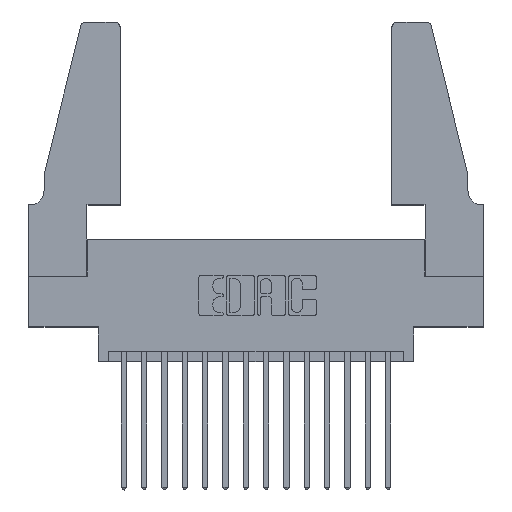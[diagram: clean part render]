
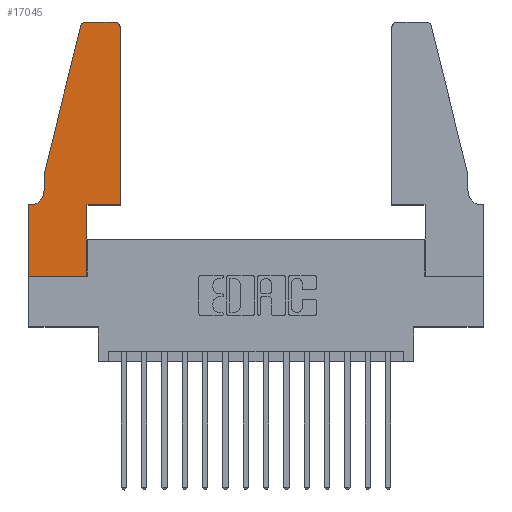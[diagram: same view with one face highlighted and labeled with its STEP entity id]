
A CAD part, top view. The second image highlights one B-rep face of the part: STEP entity #17045.
In plain terms, the highlighted planar face has unit normal (0, 0, 1).
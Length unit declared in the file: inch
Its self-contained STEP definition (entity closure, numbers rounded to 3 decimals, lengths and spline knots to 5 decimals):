
#61 = CARTESIAN_POINT ( 'NONE',  ( 0.284, 1.22, 0.37 ) ) ;
#124 = DIRECTION ( 'NONE',  ( 1., 0., 0. ) ) ;
#344 = EDGE_CURVE ( 'NONE', #13721, #15269, #12927, .T. ) ;
#364 = ORIENTED_EDGE ( 'NONE', *, *, #15349, .T. ) ;
#545 = CIRCLE ( 'NONE', #15114, 0.07 ) ;
#1067 = CARTESIAN_POINT ( 'NONE',  ( 0.2865, 0.35, 0.37 ) ) ;
#1148 = CARTESIAN_POINT ( 'NONE',  ( 0., 0., 0.37 ) ) ;
#1391 = LINE ( 'NONE', #13280, #16853 ) ;
#1486 = VECTOR ( 'NONE', #5687, 39.37008 ) ;
#1621 = VECTOR ( 'NONE', #5426, 39.37008 ) ;
#1681 = DIRECTION ( 'NONE',  ( 1., 0., 0. ) ) ;
#1689 = DIRECTION ( 'NONE',  ( -0.239, -0.971, 0. ) ) ;
#2082 = CARTESIAN_POINT ( 'NONE',  ( 0.0055, 0.42, 0.37 ) ) ;
#2215 = ORIENTED_EDGE ( 'NONE', *, *, #9709, .T. ) ;
#2290 = EDGE_CURVE ( 'NONE', #10791, #10684, #3762, .T. ) ;
#2523 = ORIENTED_EDGE ( 'NONE', *, *, #15276, .T. ) ;
#2756 = CARTESIAN_POINT ( 'NONE',  ( 0., 0., 0.37 ) ) ;
#2840 = CARTESIAN_POINT ( 'NONE',  ( 0.0755, 0.35, 0.37 ) ) ;
#2847 = ORIENTED_EDGE ( 'NONE', *, *, #7141, .T. ) ;
#3044 = CARTESIAN_POINT ( 'NONE',  ( 0.284, 1.25, 0.37 ) ) ;
#3059 = VERTEX_POINT ( 'NONE', #8273 ) ;
#3680 = ORIENTED_EDGE ( 'NONE', *, *, #344, .T. ) ;
#3704 = DIRECTION ( 'NONE',  ( 0., -1., 0. ) ) ;
#3714 = DIRECTION ( 'NONE',  ( 0., 1., 0. ) ) ;
#3762 = LINE ( 'NONE', #14663, #9138 ) ;
#3969 = CIRCLE ( 'NONE', #9717, 0.03 ) ;
#4287 = DIRECTION ( 'NONE',  ( 0., 0., 1. ) ) ;
#4327 = ORIENTED_EDGE ( 'NONE', *, *, #2290, .T. ) ;
#4371 = LINE ( 'NONE', #14840, #10973 ) ;
#5023 = CARTESIAN_POINT ( 'NONE',  ( 0.2865, 0., 0.37 ) ) ;
#5355 = VERTEX_POINT ( 'NONE', #9984 ) ;
#5426 = DIRECTION ( 'NONE',  ( 0., -1., 0. ) ) ;
#5546 = PLANE ( 'NONE',  #7440 ) ;
#5687 = DIRECTION ( 'NONE',  ( -1., 0., 0. ) ) ;
#5721 = EDGE_CURVE ( 'NONE', #15269, #3059, #1391, .T. ) ;
#6016 = FACE_OUTER_BOUND ( 'NONE', #6773, .T. ) ;
#6397 = LINE ( 'NONE', #2756, #1621 ) ;
#6705 = CIRCLE ( 'NONE', #13779, 0.03 ) ;
#6773 = EDGE_LOOP ( 'NONE', ( #4327, #2215, #14310, #13172, #14304, #364, #13648, #2847, #7161, #3680, #8427, #2523 ) ) ;
#6896 = CARTESIAN_POINT ( 'NONE',  ( 0.4205, 1.22, 0.37 ) ) ;
#6923 = DIRECTION ( 'NONE',  ( 0., 0., 1. ) ) ;
#7141 = EDGE_CURVE ( 'NONE', #8971, #10095, #11443, .T. ) ;
#7161 = ORIENTED_EDGE ( 'NONE', *, *, #11708, .T. ) ;
#7246 = LINE ( 'NONE', #1067, #13441 ) ;
#7440 = AXIS2_PLACEMENT_3D ( 'NONE', #14804, #6923, #13326 ) ;
#7501 = CARTESIAN_POINT ( 'NONE',  ( 0.0755, 0.42, 0.37 ) ) ;
#7707 = LINE ( 'NONE', #11720, #11612 ) ;
#7789 = CARTESIAN_POINT ( 'NONE',  ( 0.0755, 0.5, 0.37 ) ) ;
#7939 = DIRECTION ( 'NONE',  ( -1., 0., 0. ) ) ;
#7954 = VECTOR ( 'NONE', #1681, 39.37008 ) ;
#8019 = DIRECTION ( 'NONE',  ( 1., 0., 0. ) ) ;
#8216 = EDGE_CURVE ( 'NONE', #11096, #10961, #7707, .T. ) ;
#8273 = CARTESIAN_POINT ( 'NONE',  ( 0.4505, 1.22, 0.37 ) ) ;
#8375 = DIRECTION ( 'NONE',  ( 0., 1., 0. ) ) ;
#8427 = ORIENTED_EDGE ( 'NONE', *, *, #5721, .T. ) ;
#8853 = CARTESIAN_POINT ( 'NONE',  ( 0.2865, 0.35, 0.37 ) ) ;
#8971 = VERTEX_POINT ( 'NONE', #1148 ) ;
#9138 = VECTOR ( 'NONE', #7939, 39.37008 ) ;
#9709 = EDGE_CURVE ( 'NONE', #10684, #5355, #6705, .T. ) ;
#9717 = AXIS2_PLACEMENT_3D ( 'NONE', #6896, #4287, #16095 ) ;
#9984 = CARTESIAN_POINT ( 'NONE',  ( 0.25487, 1.22718, 0.37 ) ) ;
#10095 = VERTEX_POINT ( 'NONE', #5023 ) ;
#10684 = VERTEX_POINT ( 'NONE', #3044 ) ;
#10791 = VERTEX_POINT ( 'NONE', #11229 ) ;
#10961 = VERTEX_POINT ( 'NONE', #7501 ) ;
#10973 = VECTOR ( 'NONE', #1689, 39.37008 ) ;
#11096 = VERTEX_POINT ( 'NONE', #7789 ) ;
#11134 = CARTESIAN_POINT ( 'NONE',  ( 0., 0., 0.37 ) ) ;
#11229 = CARTESIAN_POINT ( 'NONE',  ( 0.4205, 1.25, 0.37 ) ) ;
#11230 = VERTEX_POINT ( 'NONE', #16000 ) ;
#11443 = LINE ( 'NONE', #11134, #7954 ) ;
#11612 = VECTOR ( 'NONE', #3704, 39.37008 ) ;
#11708 = EDGE_CURVE ( 'NONE', #10095, #13721, #7246, .T. ) ;
#11720 = CARTESIAN_POINT ( 'NONE',  ( 0.0755, 0.5, 0.37 ) ) ;
#11797 = CARTESIAN_POINT ( 'NONE',  ( 0.4505, 0.35, 0.37 ) ) ;
#11986 = CARTESIAN_POINT ( 'NONE',  ( 0.4505, 0.35, 0.37 ) ) ;
#12099 = VECTOR ( 'NONE', #8019, 39.37008 ) ;
#12160 = CARTESIAN_POINT ( 'NONE',  ( 0., 0.35, 0.37 ) ) ;
#12634 = DIRECTION ( 'NONE',  ( 0., 0., -1. ) ) ;
#12741 = EDGE_CURVE ( 'NONE', #13160, #8971, #6397, .T. ) ;
#12927 = LINE ( 'NONE', #11986, #12099 ) ;
#13160 = VERTEX_POINT ( 'NONE', #12160 ) ;
#13172 = ORIENTED_EDGE ( 'NONE', *, *, #8216, .T. ) ;
#13280 = CARTESIAN_POINT ( 'NONE',  ( 0.4505, 0.35, 0.37 ) ) ;
#13326 = DIRECTION ( 'NONE',  ( 1., 0., 0. ) ) ;
#13441 = VECTOR ( 'NONE', #3714, 39.37008 ) ;
#13648 = ORIENTED_EDGE ( 'NONE', *, *, #12741, .T. ) ;
#13649 = EDGE_CURVE ( 'NONE', #10961, #11230, #545, .T. ) ;
#13721 = VERTEX_POINT ( 'NONE', #8853 ) ;
#13779 = AXIS2_PLACEMENT_3D ( 'NONE', #61, #15878, #124 ) ;
#14304 = ORIENTED_EDGE ( 'NONE', *, *, #13649, .T. ) ;
#14310 = ORIENTED_EDGE ( 'NONE', *, *, #16429, .T. ) ;
#14663 = CARTESIAN_POINT ( 'NONE',  ( 0.2605, 1.25, 0.37 ) ) ;
#14804 = CARTESIAN_POINT ( 'NONE',  ( 0., 0.35, 0.37 ) ) ;
#14840 = CARTESIAN_POINT ( 'NONE',  ( 0.0755, 0.5, 0.37 ) ) ;
#14897 = LINE ( 'NONE', #2840, #1486 ) ;
#15114 = AXIS2_PLACEMENT_3D ( 'NONE', #2082, #12634, #15343 ) ;
#15269 = VERTEX_POINT ( 'NONE', #11797 ) ;
#15276 = EDGE_CURVE ( 'NONE', #3059, #10791, #3969, .T. ) ;
#15343 = DIRECTION ( 'NONE',  ( -1., 0., 0. ) ) ;
#15349 = EDGE_CURVE ( 'NONE', #11230, #13160, #14897, .T. ) ;
#15878 = DIRECTION ( 'NONE',  ( 0., 0., 1. ) ) ;
#16000 = CARTESIAN_POINT ( 'NONE',  ( 0.0055, 0.35, 0.37 ) ) ;
#16095 = DIRECTION ( 'NONE',  ( 1., 0., 0. ) ) ;
#16429 = EDGE_CURVE ( 'NONE', #5355, #11096, #4371, .T. ) ;
#16853 = VECTOR ( 'NONE', #8375, 39.37008 ) ;
#17045 = ADVANCED_FACE ( 'NONE', ( #6016 ), #5546, .T. ) ;
